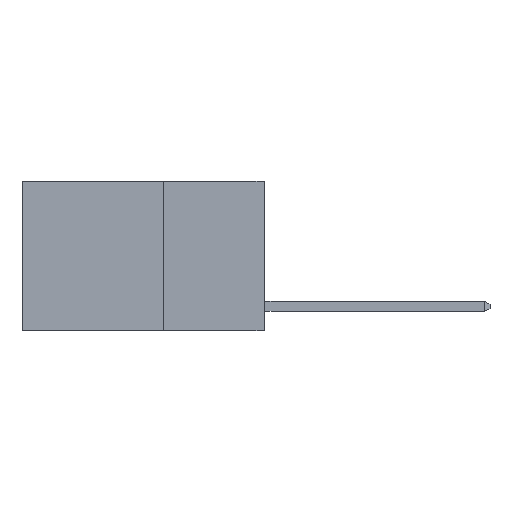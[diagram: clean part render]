
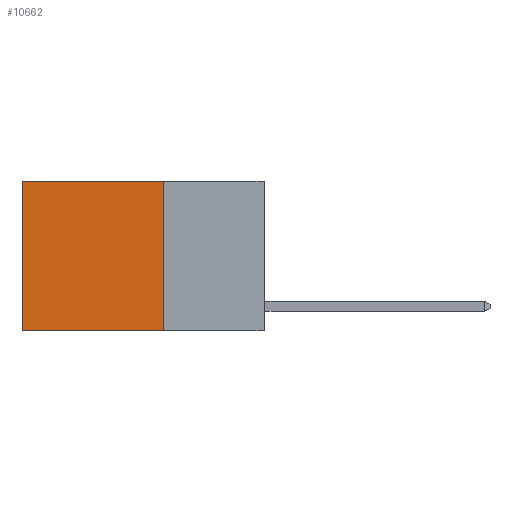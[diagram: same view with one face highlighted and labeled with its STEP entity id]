
A CAD part, left-side view. The second image highlights one B-rep face of the part: STEP entity #10662.
In plain terms, the highlighted planar face has unit normal (-1, 0, 0).
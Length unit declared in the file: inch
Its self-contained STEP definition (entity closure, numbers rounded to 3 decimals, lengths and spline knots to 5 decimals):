
#509 = VECTOR ( 'NONE', #4122, 39.37008 ) ;
#530 = ORIENTED_EDGE ( 'NONE', *, *, #10931, .F. ) ;
#684 = DIRECTION ( 'NONE',  ( 0., 0., -1. ) ) ;
#707 = CARTESIAN_POINT ( 'NONE',  ( 0.2625, 0.25, 0. ) ) ;
#1127 = AXIS2_PLACEMENT_3D ( 'NONE', #11332, #6013, #684 ) ;
#1489 = EDGE_CURVE ( 'NONE', #2376, #6516, #2882, .T. ) ;
#1541 = DIRECTION ( 'NONE',  ( 0., 0., -1. ) ) ;
#2080 = EDGE_CURVE ( 'NONE', #6516, #6667, #5909, .T. ) ;
#2376 = VERTEX_POINT ( 'NONE', #707 ) ;
#2728 = FACE_OUTER_BOUND ( 'NONE', #7119, .T. ) ;
#2882 = LINE ( 'NONE', #2992, #509 ) ;
#2992 = CARTESIAN_POINT ( 'NONE',  ( 0.2625, 0.25, 0. ) ) ;
#3058 = CARTESIAN_POINT ( 'NONE',  ( 0.2625, 0.25, 0. ) ) ;
#3666 = LINE ( 'NONE', #3058, #11001 ) ;
#4122 = DIRECTION ( 'NONE',  ( 0., 1., 0. ) ) ;
#4736 = EDGE_CURVE ( 'NONE', #2376, #8068, #3666, .T. ) ;
#4942 = LINE ( 'NONE', #10852, #11199 ) ;
#5124 = PLANE ( 'NONE',  #1127 ) ;
#5909 = LINE ( 'NONE', #9595, #8019 ) ;
#6013 = DIRECTION ( 'NONE',  ( 1., 0., 0. ) ) ;
#6516 = VERTEX_POINT ( 'NONE', #7507 ) ;
#6667 = VERTEX_POINT ( 'NONE', #9472 ) ;
#7119 = EDGE_LOOP ( 'NONE', ( #8980, #530, #10375, #7301 ) ) ;
#7301 = ORIENTED_EDGE ( 'NONE', *, *, #1489, .T. ) ;
#7507 = CARTESIAN_POINT ( 'NONE',  ( 0.2625, 0.6, 0. ) ) ;
#8019 = VECTOR ( 'NONE', #1541, 39.37008 ) ;
#8068 = VERTEX_POINT ( 'NONE', #11338 ) ;
#8980 = ORIENTED_EDGE ( 'NONE', *, *, #2080, .T. ) ;
#9060 = DIRECTION ( 'NONE',  ( 0., 1., 0. ) ) ;
#9266 = DIRECTION ( 'NONE',  ( 0., 0., -1. ) ) ;
#9472 = CARTESIAN_POINT ( 'NONE',  ( 0.2625, 0.6, -0.37 ) ) ;
#9595 = CARTESIAN_POINT ( 'NONE',  ( 0.2625, 0.6, 0. ) ) ;
#10375 = ORIENTED_EDGE ( 'NONE', *, *, #4736, .F. ) ;
#10662 = ADVANCED_FACE ( 'NONE', ( #2728 ), #5124, .F. ) ;
#10852 = CARTESIAN_POINT ( 'NONE',  ( 0.2625, 0.25, -0.37 ) ) ;
#10931 = EDGE_CURVE ( 'NONE', #8068, #6667, #4942, .T. ) ;
#11001 = VECTOR ( 'NONE', #9266, 39.37008 ) ;
#11199 = VECTOR ( 'NONE', #9060, 39.37008 ) ;
#11332 = CARTESIAN_POINT ( 'NONE',  ( 0.2625, 0.25, 0. ) ) ;
#11338 = CARTESIAN_POINT ( 'NONE',  ( 0.2625, 0.25, -0.37 ) ) ;
